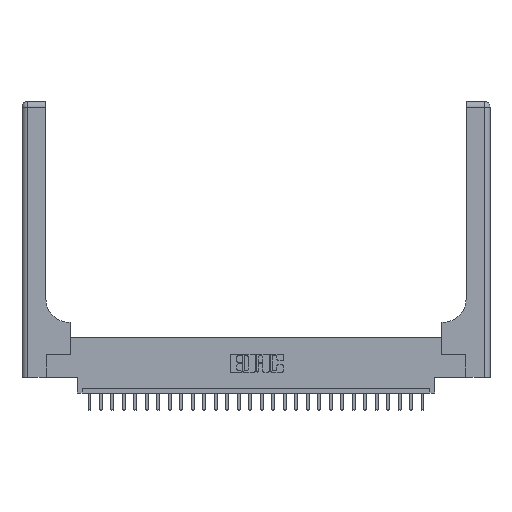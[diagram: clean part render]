
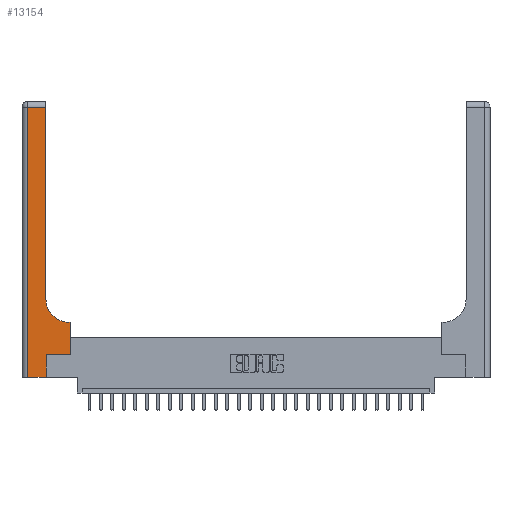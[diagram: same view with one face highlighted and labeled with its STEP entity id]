
A CAD part, top view. The second image highlights one B-rep face of the part: STEP entity #13154.
In plain terms, the highlighted planar face has unit normal (0, 0, 1).
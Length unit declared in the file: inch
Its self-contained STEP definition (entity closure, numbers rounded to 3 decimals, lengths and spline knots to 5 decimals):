
#301 = VECTOR ( 'NONE', #17737, 39.37008 ) ;
#541 = ORIENTED_EDGE ( 'NONE', *, *, #11144, .T. ) ;
#980 = CARTESIAN_POINT ( 'NONE',  ( 0.528, 0.6, 0.37 ) ) ;
#1038 = ORIENTED_EDGE ( 'NONE', *, *, #12825, .T. ) ;
#1352 = ORIENTED_EDGE ( 'NONE', *, *, #15847, .T. ) ;
#1399 = AXIS2_PLACEMENT_3D ( 'NONE', #1926, #7825, #9834 ) ;
#1926 = CARTESIAN_POINT ( 'NONE',  ( 0., 3., 0.37 ) ) ;
#2081 = CARTESIAN_POINT ( 'NONE',  ( 0.265, 0.25, 0.37 ) ) ;
#2126 = CARTESIAN_POINT ( 'NONE',  ( 0.26, 0.85, 0.37 ) ) ;
#2147 = VERTEX_POINT ( 'NONE', #6041 ) ;
#2459 = DIRECTION ( 'NONE',  ( 1., 0., 0. ) ) ;
#2475 = CARTESIAN_POINT ( 'NONE',  ( 0.265, 0., 0.37 ) ) ;
#3055 = EDGE_CURVE ( 'NONE', #4964, #16922, #6942, .T. ) ;
#3191 = LINE ( 'NONE', #15434, #23664 ) ;
#3203 = EDGE_CURVE ( 'NONE', #16922, #11258, #3191, .T. ) ;
#3277 = LINE ( 'NONE', #2475, #9813 ) ;
#3759 = CARTESIAN_POINT ( 'NONE',  ( 0.26, 0.6, 0.37 ) ) ;
#3924 = LINE ( 'NONE', #6645, #5478 ) ;
#4001 = ORIENTED_EDGE ( 'NONE', *, *, #19009, .T. ) ;
#4182 = VECTOR ( 'NONE', #4540, 39.37008 ) ;
#4427 = VECTOR ( 'NONE', #22668, 39.37008 ) ;
#4540 = DIRECTION ( 'NONE',  ( -1., 0., 0. ) ) ;
#4636 = ORIENTED_EDGE ( 'NONE', *, *, #21891, .T. ) ;
#4951 = CARTESIAN_POINT ( 'NONE',  ( 0.528, 0.25, 0.37 ) ) ;
#4964 = VERTEX_POINT ( 'NONE', #7956 ) ;
#5055 = CARTESIAN_POINT ( 'NONE',  ( 0.528, 0.25, 0.37 ) ) ;
#5392 = CARTESIAN_POINT ( 'NONE',  ( 0.265, 0., 0.37 ) ) ;
#5478 = VECTOR ( 'NONE', #20512, 39.37008 ) ;
#5667 = VERTEX_POINT ( 'NONE', #2081 ) ;
#6041 = CARTESIAN_POINT ( 'NONE',  ( 0.06, 0., 0.37 ) ) ;
#6266 = ORIENTED_EDGE ( 'NONE', *, *, #3203, .T. ) ;
#6645 = CARTESIAN_POINT ( 'NONE',  ( 0.265, 0.25, 0.37 ) ) ;
#6942 = CIRCLE ( 'NONE', #17286, 0.25 ) ;
#7108 = ORIENTED_EDGE ( 'NONE', *, *, #11896, .T. ) ;
#7225 = DIRECTION ( 'NONE',  ( 0., 1., 0. ) ) ;
#7524 = DIRECTION ( 'NONE',  ( 0., 1., 0. ) ) ;
#7825 = DIRECTION ( 'NONE',  ( 0., 0., -1. ) ) ;
#7956 = CARTESIAN_POINT ( 'NONE',  ( 0.51, 0.6, 0.37 ) ) ;
#8268 = CARTESIAN_POINT ( 'NONE',  ( 0.06, 3., 0.37 ) ) ;
#8369 = LINE ( 'NONE', #25102, #301 ) ;
#8550 = CARTESIAN_POINT ( 'NONE',  ( 0.51, 0.85, 0.37 ) ) ;
#8661 = DIRECTION ( 'NONE',  ( 0., 1., 0. ) ) ;
#9664 = LINE ( 'NONE', #4951, #19584 ) ;
#9751 = LINE ( 'NONE', #8268, #4427 ) ;
#9813 = VECTOR ( 'NONE', #8661, 39.37008 ) ;
#9834 = DIRECTION ( 'NONE',  ( -1., 0., 0. ) ) ;
#10392 = CARTESIAN_POINT ( 'NONE',  ( 0.06, 2.94, 0.37 ) ) ;
#11017 = VERTEX_POINT ( 'NONE', #980 ) ;
#11144 = EDGE_CURVE ( 'NONE', #5667, #15222, #3924, .T. ) ;
#11258 = VERTEX_POINT ( 'NONE', #23444 ) ;
#11896 = EDGE_CURVE ( 'NONE', #14214, #5667, #3277, .T. ) ;
#12704 = DIRECTION ( 'NONE',  ( 0., 0., -1. ) ) ;
#12825 = EDGE_CURVE ( 'NONE', #2147, #14214, #24938, .T. ) ;
#13154 = ADVANCED_FACE ( 'NONE', ( #21794 ), #19716, .F. ) ;
#14097 = ORIENTED_EDGE ( 'NONE', *, *, #3055, .T. ) ;
#14214 = VERTEX_POINT ( 'NONE', #5392 ) ;
#15063 = VERTEX_POINT ( 'NONE', #10392 ) ;
#15087 = LINE ( 'NONE', #3759, #4182 ) ;
#15222 = VERTEX_POINT ( 'NONE', #5055 ) ;
#15434 = CARTESIAN_POINT ( 'NONE',  ( 0.26, 3., 0.37 ) ) ;
#15847 = EDGE_CURVE ( 'NONE', #11258, #15063, #8369, .T. ) ;
#16922 = VERTEX_POINT ( 'NONE', #2126 ) ;
#17286 = AXIS2_PLACEMENT_3D ( 'NONE', #8550, #12704, #24894 ) ;
#17661 = EDGE_CURVE ( 'NONE', #11017, #4964, #15087, .T. ) ;
#17737 = DIRECTION ( 'NONE',  ( -1., 0., 0. ) ) ;
#18273 = CARTESIAN_POINT ( 'NONE',  ( 0., 0., 0.37 ) ) ;
#19009 = EDGE_CURVE ( 'NONE', #15063, #2147, #9751, .T. ) ;
#19584 = VECTOR ( 'NONE', #7225, 39.37008 ) ;
#19716 = PLANE ( 'NONE',  #1399 ) ;
#20512 = DIRECTION ( 'NONE',  ( 1., 0., 0. ) ) ;
#21794 = FACE_OUTER_BOUND ( 'NONE', #23084, .T. ) ;
#21891 = EDGE_CURVE ( 'NONE', #15222, #11017, #9664, .T. ) ;
#22668 = DIRECTION ( 'NONE',  ( 0., -1., 0. ) ) ;
#23084 = EDGE_LOOP ( 'NONE', ( #6266, #1352, #4001, #1038, #7108, #541, #4636, #23955, #14097 ) ) ;
#23444 = CARTESIAN_POINT ( 'NONE',  ( 0.26, 2.94, 0.37 ) ) ;
#23664 = VECTOR ( 'NONE', #7524, 39.37008 ) ;
#23955 = ORIENTED_EDGE ( 'NONE', *, *, #17661, .T. ) ;
#24894 = DIRECTION ( 'NONE',  ( 1., 0., 0. ) ) ;
#24938 = LINE ( 'NONE', #18273, #25557 ) ;
#25102 = CARTESIAN_POINT ( 'NONE',  ( 0., 2.94, 0.37 ) ) ;
#25557 = VECTOR ( 'NONE', #2459, 39.37008 ) ;
